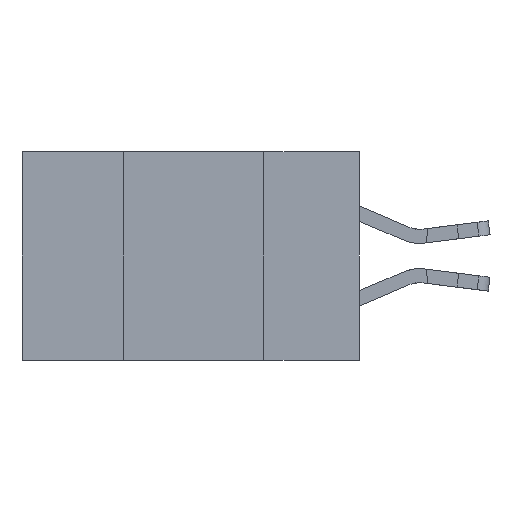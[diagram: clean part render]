
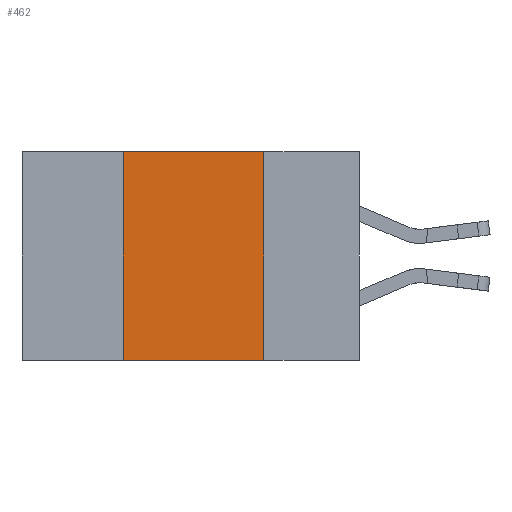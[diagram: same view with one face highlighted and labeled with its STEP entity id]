
A CAD part, left-side view. The second image highlights one B-rep face of the part: STEP entity #462.
In plain terms, the highlighted planar face has unit normal (-1, 0, 0).
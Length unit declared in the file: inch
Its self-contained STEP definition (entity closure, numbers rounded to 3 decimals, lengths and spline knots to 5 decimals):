
#462 = ADVANCED_FACE ( 'NONE', ( #2533 ), #10134, .F. ) ;
#518 = ORIENTED_EDGE ( 'NONE', *, *, #8455, .T. ) ;
#577 = ORIENTED_EDGE ( 'NONE', *, *, #8785, .F. ) ;
#1270 = EDGE_LOOP ( 'NONE', ( #577, #4288, #13556, #518 ) ) ;
#2302 = CARTESIAN_POINT ( 'NONE',  ( 0., 0.6, 0. ) ) ;
#2510 = LINE ( 'NONE', #5273, #5316 ) ;
#2533 = FACE_OUTER_BOUND ( 'NONE', #1270, .T. ) ;
#3413 = LINE ( 'NONE', #16748, #3855 ) ;
#3789 = CARTESIAN_POINT ( 'NONE',  ( 0., 0.6, -0.37 ) ) ;
#3855 = VECTOR ( 'NONE', #14002, 39.37008 ) ;
#4288 = ORIENTED_EDGE ( 'NONE', *, *, #4844, .F. ) ;
#4844 = EDGE_CURVE ( 'NONE', #16196, #15325, #17584, .T. ) ;
#5273 = CARTESIAN_POINT ( 'NONE',  ( 0., 0.42, 0. ) ) ;
#5316 = VECTOR ( 'NONE', #14805, 39.37008 ) ;
#5384 = LINE ( 'NONE', #3789, #12651 ) ;
#5850 = CARTESIAN_POINT ( 'NONE',  ( 0., 0.6, 0. ) ) ;
#5906 = DIRECTION ( 'NONE',  ( 1., 0., 0. ) ) ;
#6748 = VECTOR ( 'NONE', #16722, 39.37008 ) ;
#8110 = DIRECTION ( 'NONE',  ( 0., 0., -1. ) ) ;
#8455 = EDGE_CURVE ( 'NONE', #9665, #16324, #5384, .T. ) ;
#8785 = EDGE_CURVE ( 'NONE', #15325, #16324, #3413, .T. ) ;
#9464 = CARTESIAN_POINT ( 'NONE',  ( 0., 0.42, -0.37 ) ) ;
#9665 = VERTEX_POINT ( 'NONE', #9464 ) ;
#10134 = PLANE ( 'NONE',  #13685 ) ;
#11524 = EDGE_CURVE ( 'NONE', #9665, #16196, #2510, .T. ) ;
#11998 = DIRECTION ( 'NONE',  ( 0., -1., 0. ) ) ;
#12651 = VECTOR ( 'NONE', #11998, 39.37008 ) ;
#12975 = CARTESIAN_POINT ( 'NONE',  ( 0., 0.42, 0. ) ) ;
#13556 = ORIENTED_EDGE ( 'NONE', *, *, #11524, .F. ) ;
#13656 = CARTESIAN_POINT ( 'NONE',  ( 0., 0.17, 0. ) ) ;
#13685 = AXIS2_PLACEMENT_3D ( 'NONE', #2302, #5906, #8110 ) ;
#14002 = DIRECTION ( 'NONE',  ( 0., 0., -1. ) ) ;
#14640 = CARTESIAN_POINT ( 'NONE',  ( 0., 0.17, -0.37 ) ) ;
#14805 = DIRECTION ( 'NONE',  ( 0., 0., 1. ) ) ;
#15325 = VERTEX_POINT ( 'NONE', #13656 ) ;
#16196 = VERTEX_POINT ( 'NONE', #12975 ) ;
#16324 = VERTEX_POINT ( 'NONE', #14640 ) ;
#16722 = DIRECTION ( 'NONE',  ( 0., -1., 0. ) ) ;
#16748 = CARTESIAN_POINT ( 'NONE',  ( 0., 0.17, 0. ) ) ;
#17584 = LINE ( 'NONE', #5850, #6748 ) ;
